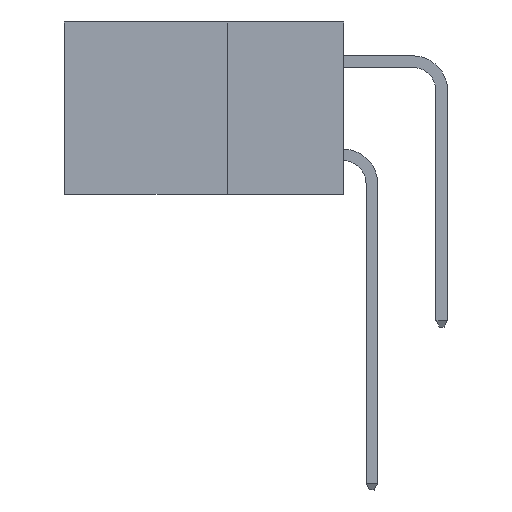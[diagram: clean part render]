
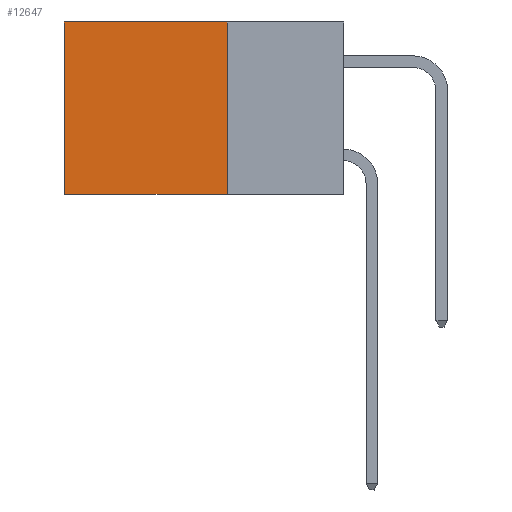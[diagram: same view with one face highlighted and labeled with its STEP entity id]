
A CAD part, left-side view. The second image highlights one B-rep face of the part: STEP entity #12647.
In plain terms, the highlighted planar face has unit normal (-1, 0, 0).
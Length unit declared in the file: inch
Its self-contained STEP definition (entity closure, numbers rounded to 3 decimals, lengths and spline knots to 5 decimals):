
#46 = LINE ( 'NONE', #12462, #6723 ) ;
#137 = FACE_OUTER_BOUND ( 'NONE', #3763, .T. ) ;
#581 = VECTOR ( 'NONE', #11056, 39.37008 ) ;
#1531 = DIRECTION ( 'NONE',  ( 0., 0., -1. ) ) ;
#2320 = VERTEX_POINT ( 'NONE', #15742 ) ;
#2358 = ORIENTED_EDGE ( 'NONE', *, *, #15364, .F. ) ;
#2516 = EDGE_CURVE ( 'NONE', #10268, #2320, #6675, .T. ) ;
#3602 = ORIENTED_EDGE ( 'NONE', *, *, #8572, .T. ) ;
#3763 = EDGE_LOOP ( 'NONE', ( #3602, #6375, #2358, #5373 ) ) ;
#3937 = VECTOR ( 'NONE', #18217, 39.37008 ) ;
#5373 = ORIENTED_EDGE ( 'NONE', *, *, #2516, .T. ) ;
#6342 = DIRECTION ( 'NONE',  ( 1., 0., 0. ) ) ;
#6375 = ORIENTED_EDGE ( 'NONE', *, *, #11228, .F. ) ;
#6675 = LINE ( 'NONE', #12883, #581 ) ;
#6723 = VECTOR ( 'NONE', #10524, 39.37008 ) ;
#7784 = DIRECTION ( 'NONE',  ( 0., 0., -1. ) ) ;
#8572 = EDGE_CURVE ( 'NONE', #2320, #11199, #12001, .T. ) ;
#10268 = VERTEX_POINT ( 'NONE', #16006 ) ;
#10524 = DIRECTION ( 'NONE',  ( 0., 1., 0. ) ) ;
#10837 = PLANE ( 'NONE',  #12291 ) ;
#10921 = VERTEX_POINT ( 'NONE', #14424 ) ;
#11056 = DIRECTION ( 'NONE',  ( 0., 1., 0. ) ) ;
#11199 = VERTEX_POINT ( 'NONE', #15330 ) ;
#11228 = EDGE_CURVE ( 'NONE', #10921, #11199, #46, .T. ) ;
#12001 = LINE ( 'NONE', #19553, #3937 ) ;
#12291 = AXIS2_PLACEMENT_3D ( 'NONE', #15523, #6342, #7784 ) ;
#12462 = CARTESIAN_POINT ( 'NONE',  ( 0.2615, 0.25, -0.37 ) ) ;
#12647 = ADVANCED_FACE ( 'NONE', ( #137 ), #10837, .F. ) ;
#12883 = CARTESIAN_POINT ( 'NONE',  ( 0.2615, 0.25, 0. ) ) ;
#14424 = CARTESIAN_POINT ( 'NONE',  ( 0.2615, 0.25, -0.37 ) ) ;
#15330 = CARTESIAN_POINT ( 'NONE',  ( 0.2615, 0.6, -0.37 ) ) ;
#15364 = EDGE_CURVE ( 'NONE', #10268, #10921, #18728, .T. ) ;
#15523 = CARTESIAN_POINT ( 'NONE',  ( 0.2615, 0.25, -0.37 ) ) ;
#15742 = CARTESIAN_POINT ( 'NONE',  ( 0.2615, 0.6, 0. ) ) ;
#16006 = CARTESIAN_POINT ( 'NONE',  ( 0.2615, 0.25, 0. ) ) ;
#17014 = CARTESIAN_POINT ( 'NONE',  ( 0.2615, 0.25, -0.37 ) ) ;
#18217 = DIRECTION ( 'NONE',  ( 0., 0., -1. ) ) ;
#18556 = VECTOR ( 'NONE', #1531, 39.37008 ) ;
#18728 = LINE ( 'NONE', #17014, #18556 ) ;
#19553 = CARTESIAN_POINT ( 'NONE',  ( 0.2615, 0.6, -0.37 ) ) ;
